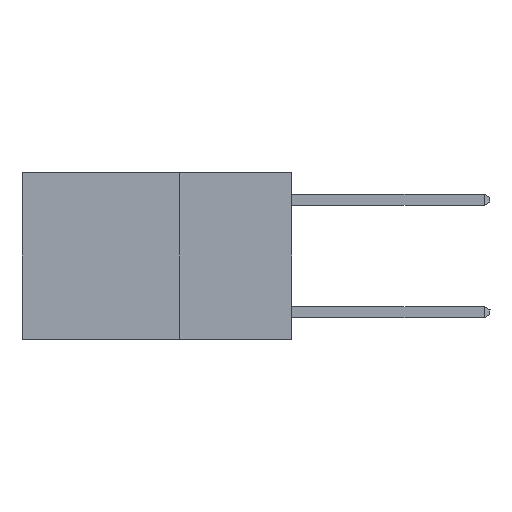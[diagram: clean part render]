
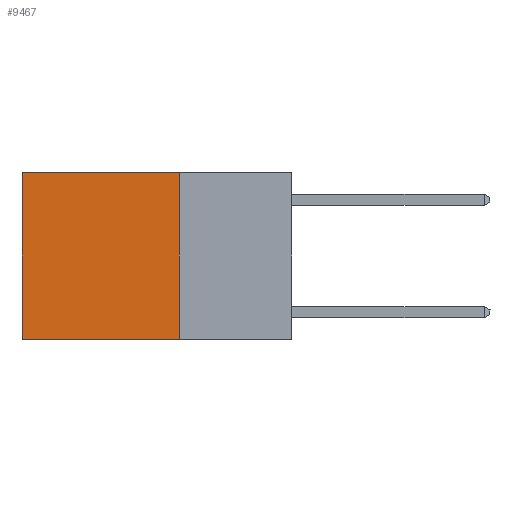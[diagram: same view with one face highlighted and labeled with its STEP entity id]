
A CAD part, left-side view. The second image highlights one B-rep face of the part: STEP entity #9467.
In plain terms, the highlighted planar face has unit normal (-1, 0, 0).
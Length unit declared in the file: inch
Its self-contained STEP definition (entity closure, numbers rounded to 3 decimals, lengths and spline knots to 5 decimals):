
#108 = CARTESIAN_POINT ( 'NONE',  ( 0.2625, 0.6, 0. ) ) ;
#234 = EDGE_CURVE ( 'NONE', #7992, #9610, #695, .T. ) ;
#695 = LINE ( 'NONE', #8613, #4767 ) ;
#858 = ORIENTED_EDGE ( 'NONE', *, *, #2000, .T. ) ;
#933 = DIRECTION ( 'NONE',  ( 0., 0., -1. ) ) ;
#1148 = VECTOR ( 'NONE', #933, 39.37008 ) ;
#1180 = EDGE_CURVE ( 'NONE', #7992, #7810, #2070, .T. ) ;
#1948 = CARTESIAN_POINT ( 'NONE',  ( 0.2625, 0.6, -0.37 ) ) ;
#2000 = EDGE_CURVE ( 'NONE', #9610, #2889, #7623, .T. ) ;
#2070 = LINE ( 'NONE', #3175, #6395 ) ;
#2762 = CARTESIAN_POINT ( 'NONE',  ( 0.2625, 0.25, -0.37 ) ) ;
#2889 = VERTEX_POINT ( 'NONE', #1948 ) ;
#3166 = DIRECTION ( 'NONE',  ( 0., 0., -1. ) ) ;
#3175 = CARTESIAN_POINT ( 'NONE',  ( 0.2625, 0.25, 0. ) ) ;
#3938 = LINE ( 'NONE', #8885, #7990 ) ;
#4089 = DIRECTION ( 'NONE',  ( 0., 0., -1. ) ) ;
#4767 = VECTOR ( 'NONE', #8625, 39.37008 ) ;
#4836 = DIRECTION ( 'NONE',  ( 0., 1., 0. ) ) ;
#5697 = ORIENTED_EDGE ( 'NONE', *, *, #1180, .F. ) ;
#6395 = VECTOR ( 'NONE', #3166, 39.37008 ) ;
#6481 = CARTESIAN_POINT ( 'NONE',  ( 0.2625, 0.25, 0. ) ) ;
#7044 = CARTESIAN_POINT ( 'NONE',  ( 0.2625, 0.25, 0. ) ) ;
#7332 = ORIENTED_EDGE ( 'NONE', *, *, #7562, .F. ) ;
#7562 = EDGE_CURVE ( 'NONE', #7810, #2889, #3938, .T. ) ;
#7623 = LINE ( 'NONE', #108, #1148 ) ;
#7810 = VERTEX_POINT ( 'NONE', #2762 ) ;
#7990 = VECTOR ( 'NONE', #4836, 39.37008 ) ;
#7992 = VERTEX_POINT ( 'NONE', #7044 ) ;
#8077 = ORIENTED_EDGE ( 'NONE', *, *, #234, .T. ) ;
#8119 = PLANE ( 'NONE',  #9084 ) ;
#8263 = CARTESIAN_POINT ( 'NONE',  ( 0.2625, 0.6, 0. ) ) ;
#8613 = CARTESIAN_POINT ( 'NONE',  ( 0.2625, 0.25, 0. ) ) ;
#8625 = DIRECTION ( 'NONE',  ( 0., 1., 0. ) ) ;
#8885 = CARTESIAN_POINT ( 'NONE',  ( 0.2625, 0.25, -0.37 ) ) ;
#8976 = DIRECTION ( 'NONE',  ( 1., 0., 0. ) ) ;
#9084 = AXIS2_PLACEMENT_3D ( 'NONE', #6481, #8976, #4089 ) ;
#9467 = ADVANCED_FACE ( 'NONE', ( #10028 ), #8119, .F. ) ;
#9610 = VERTEX_POINT ( 'NONE', #8263 ) ;
#10028 = FACE_OUTER_BOUND ( 'NONE', #10178, .T. ) ;
#10178 = EDGE_LOOP ( 'NONE', ( #858, #7332, #5697, #8077 ) ) ;
